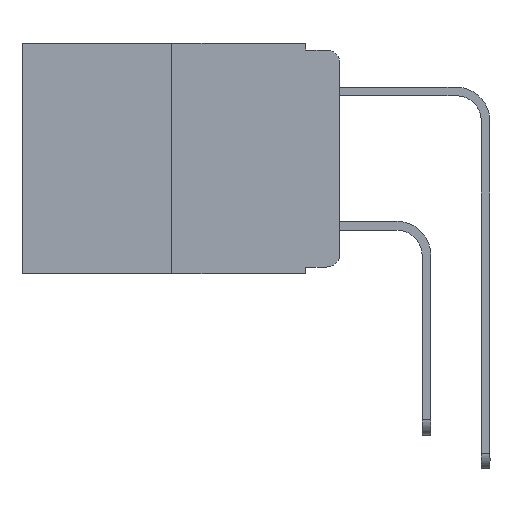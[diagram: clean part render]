
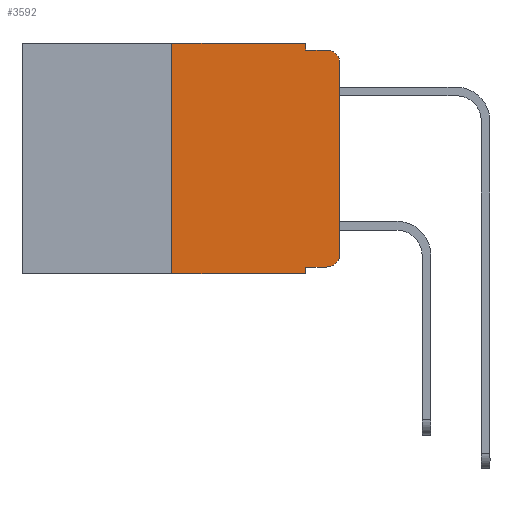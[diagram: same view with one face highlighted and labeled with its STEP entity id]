
A CAD part, left-side view. The second image highlights one B-rep face of the part: STEP entity #3592.
In plain terms, the highlighted planar face has unit normal (-1, 0, 0).
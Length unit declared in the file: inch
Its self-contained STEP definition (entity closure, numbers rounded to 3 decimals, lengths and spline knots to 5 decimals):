
#58 = CARTESIAN_POINT ( 'NONE',  ( 0., 0.051, -0.333 ) ) ;
#79 = ORIENTED_EDGE ( 'NONE', *, *, #15407, .F. ) ;
#377 = DIRECTION ( 'NONE',  ( 0., 0., -1. ) ) ;
#519 = VECTOR ( 'NONE', #22517, 39.37008 ) ;
#617 = EDGE_LOOP ( 'NONE', ( #8350, #4153, #6131, #1174, #8708, #11608, #13389, #79, #16863, #1860 ) ) ;
#811 = VECTOR ( 'NONE', #4502, 39.37008 ) ;
#1174 = ORIENTED_EDGE ( 'NONE', *, *, #6194, .F. ) ;
#1251 = VECTOR ( 'NONE', #13685, 39.37008 ) ;
#1385 = DIRECTION ( 'NONE',  ( 0., -1., 0. ) ) ;
#1420 = AXIS2_PLACEMENT_3D ( 'NONE', #12669, #17717, #10708 ) ;
#1491 = AXIS2_PLACEMENT_3D ( 'NONE', #20740, #19023, #377 ) ;
#1514 = LINE ( 'NONE', #12121, #19828 ) ;
#1860 = ORIENTED_EDGE ( 'NONE', *, *, #8743, .T. ) ;
#2032 = DIRECTION ( 'NONE',  ( 0., 0., -1. ) ) ;
#2446 = EDGE_CURVE ( 'NONE', #17182, #12665, #16049, .T. ) ;
#2450 = LINE ( 'NONE', #16499, #4028 ) ;
#2670 = CARTESIAN_POINT ( 'NONE',  ( 0., 0.473, -0.343 ) ) ;
#2736 = CARTESIAN_POINT ( 'NONE',  ( 0., 0.25, 0. ) ) ;
#2970 = LINE ( 'NONE', #20772, #519 ) ;
#3592 = ADVANCED_FACE ( 'NONE', ( #13763 ), #8570, .F. ) ;
#4028 = VECTOR ( 'NONE', #19819, 39.37008 ) ;
#4153 = ORIENTED_EDGE ( 'NONE', *, *, #4507, .T. ) ;
#4502 = DIRECTION ( 'NONE',  ( 0., -1., 0. ) ) ;
#4507 = EDGE_CURVE ( 'NONE', #14280, #10114, #13902, .T. ) ;
#4676 = LINE ( 'NONE', #6630, #1251 ) ;
#4776 = VERTEX_POINT ( 'NONE', #20423 ) ;
#4908 = CARTESIAN_POINT ( 'NONE',  ( 0., 0., 0. ) ) ;
#5261 = CARTESIAN_POINT ( 'NONE',  ( 0., 0.02, -0.03 ) ) ;
#5341 = VECTOR ( 'NONE', #18943, 39.37008 ) ;
#5433 = CARTESIAN_POINT ( 'NONE',  ( 0., 0.051, -0.343 ) ) ;
#6115 = EDGE_CURVE ( 'NONE', #14088, #22634, #2970, .T. ) ;
#6131 = ORIENTED_EDGE ( 'NONE', *, *, #17235, .F. ) ;
#6194 = EDGE_CURVE ( 'NONE', #4776, #14383, #4676, .T. ) ;
#6630 = CARTESIAN_POINT ( 'NONE',  ( 0., 0.051, 0. ) ) ;
#8350 = ORIENTED_EDGE ( 'NONE', *, *, #10863, .T. ) ;
#8364 = VERTEX_POINT ( 'NONE', #5433 ) ;
#8553 = EDGE_CURVE ( 'NONE', #22634, #4776, #12102, .T. ) ;
#8570 = PLANE ( 'NONE',  #1491 ) ;
#8708 = ORIENTED_EDGE ( 'NONE', *, *, #8553, .F. ) ;
#8743 = EDGE_CURVE ( 'NONE', #12665, #17130, #11360, .T. ) ;
#8800 = DIRECTION ( 'NONE',  ( 0., -1., 0. ) ) ;
#10114 = VERTEX_POINT ( 'NONE', #20228 ) ;
#10708 = DIRECTION ( 'NONE',  ( 0., 0., -1. ) ) ;
#10863 = EDGE_CURVE ( 'NONE', #17130, #14280, #12053, .T. ) ;
#11360 = CIRCLE ( 'NONE', #1420, 0.02 ) ;
#11608 = ORIENTED_EDGE ( 'NONE', *, *, #6115, .F. ) ;
#11766 = CARTESIAN_POINT ( 'NONE',  ( 0., 0.473, 0. ) ) ;
#12053 = LINE ( 'NONE', #4908, #5341 ) ;
#12054 = AXIS2_PLACEMENT_3D ( 'NONE', #5261, #12297, #2032 ) ;
#12102 = LINE ( 'NONE', #11766, #20092 ) ;
#12121 = CARTESIAN_POINT ( 'NONE',  ( 0., 0.051, -0.01 ) ) ;
#12297 = DIRECTION ( 'NONE',  ( -1., 0., 0. ) ) ;
#12665 = VERTEX_POINT ( 'NONE', #21518 ) ;
#12669 = CARTESIAN_POINT ( 'NONE',  ( 0., 0.02, -0.313 ) ) ;
#13028 = CARTESIAN_POINT ( 'NONE',  ( 0., 0.25, -0.343 ) ) ;
#13389 = ORIENTED_EDGE ( 'NONE', *, *, #18884, .T. ) ;
#13685 = DIRECTION ( 'NONE',  ( 0., 0., -1. ) ) ;
#13763 = FACE_OUTER_BOUND ( 'NONE', #617, .T. ) ;
#13902 = CIRCLE ( 'NONE', #12054, 0.02 ) ;
#14088 = VERTEX_POINT ( 'NONE', #13028 ) ;
#14279 = CARTESIAN_POINT ( 'NONE',  ( 0., 0.051, -0.01 ) ) ;
#14280 = VERTEX_POINT ( 'NONE', #20578 ) ;
#14383 = VERTEX_POINT ( 'NONE', #14279 ) ;
#15357 = CARTESIAN_POINT ( 'NONE',  ( 0., 0.051, -0.333 ) ) ;
#15407 = EDGE_CURVE ( 'NONE', #17182, #8364, #2450, .T. ) ;
#16049 = LINE ( 'NONE', #58, #21287 ) ;
#16499 = CARTESIAN_POINT ( 'NONE',  ( 0., 0.051, 0. ) ) ;
#16863 = ORIENTED_EDGE ( 'NONE', *, *, #2446, .T. ) ;
#17130 = VERTEX_POINT ( 'NONE', #22253 ) ;
#17182 = VERTEX_POINT ( 'NONE', #15357 ) ;
#17235 = EDGE_CURVE ( 'NONE', #14383, #10114, #1514, .T. ) ;
#17717 = DIRECTION ( 'NONE',  ( -1., 0., 0. ) ) ;
#18429 = LINE ( 'NONE', #2670, #811 ) ;
#18884 = EDGE_CURVE ( 'NONE', #14088, #8364, #18429, .T. ) ;
#18943 = DIRECTION ( 'NONE',  ( 0., 0., 1. ) ) ;
#19023 = DIRECTION ( 'NONE',  ( 1., 0., 0. ) ) ;
#19128 = DIRECTION ( 'NONE',  ( 0., -1., 0. ) ) ;
#19819 = DIRECTION ( 'NONE',  ( 0., 0., -1. ) ) ;
#19828 = VECTOR ( 'NONE', #19128, 39.37008 ) ;
#20092 = VECTOR ( 'NONE', #1385, 39.37008 ) ;
#20228 = CARTESIAN_POINT ( 'NONE',  ( 0., 0.02, -0.01 ) ) ;
#20423 = CARTESIAN_POINT ( 'NONE',  ( 0., 0.051, 0. ) ) ;
#20578 = CARTESIAN_POINT ( 'NONE',  ( 0., 0., -0.03 ) ) ;
#20740 = CARTESIAN_POINT ( 'NONE',  ( 0., 0.473, 0. ) ) ;
#20772 = CARTESIAN_POINT ( 'NONE',  ( 0., 0.25, 0. ) ) ;
#21287 = VECTOR ( 'NONE', #8800, 39.37008 ) ;
#21518 = CARTESIAN_POINT ( 'NONE',  ( 0., 0.02, -0.333 ) ) ;
#22253 = CARTESIAN_POINT ( 'NONE',  ( 0., 0., -0.313 ) ) ;
#22517 = DIRECTION ( 'NONE',  ( 0., 0., 1. ) ) ;
#22634 = VERTEX_POINT ( 'NONE', #2736 ) ;
